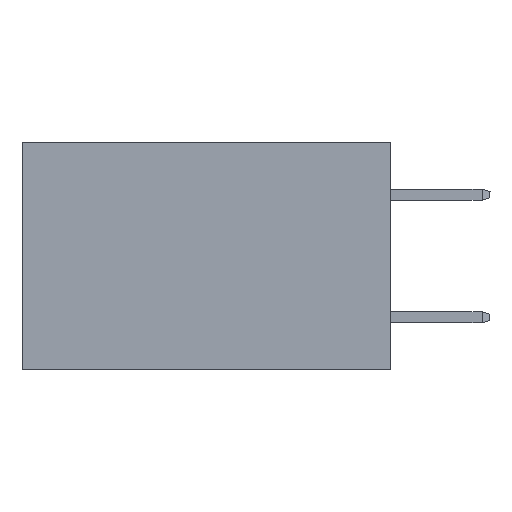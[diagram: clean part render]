
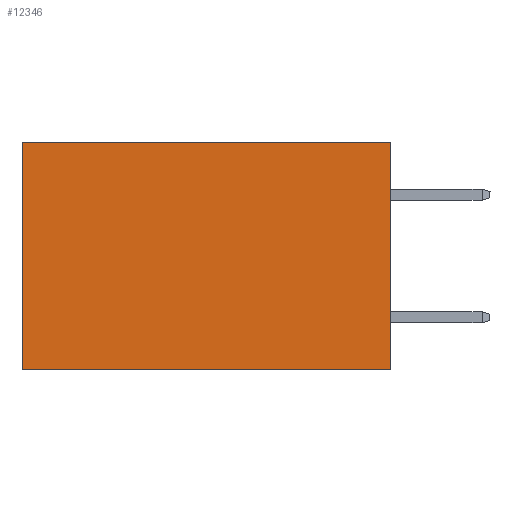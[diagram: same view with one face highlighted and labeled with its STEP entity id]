
A CAD part, left-side view. The second image highlights one B-rep face of the part: STEP entity #12346.
In plain terms, the highlighted planar face has unit normal (-1, 0, 0).
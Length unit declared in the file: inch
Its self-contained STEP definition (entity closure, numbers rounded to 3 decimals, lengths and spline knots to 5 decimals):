
#1113 = VERTEX_POINT ( 'NONE', #32478 ) ;
#1976 = VERTEX_POINT ( 'NONE', #24686 ) ;
#2902 = VECTOR ( 'NONE', #20083, 39.37008 ) ;
#5426 = CARTESIAN_POINT ( 'NONE',  ( 0.2875, 0.6, 0. ) ) ;
#5568 = DIRECTION ( 'NONE',  ( 0., 0., -1. ) ) ;
#6611 = EDGE_CURVE ( 'NONE', #1113, #8995, #24639, .T. ) ;
#7061 = DIRECTION ( 'NONE',  ( 0., 0., -1. ) ) ;
#8003 = LINE ( 'NONE', #25964, #29799 ) ;
#8931 = CARTESIAN_POINT ( 'NONE',  ( 0.2875, 0., 0. ) ) ;
#8995 = VERTEX_POINT ( 'NONE', #32847 ) ;
#9160 = EDGE_CURVE ( 'NONE', #16201, #8995, #28590, .T. ) ;
#9672 = EDGE_CURVE ( 'NONE', #1976, #1113, #33399, .T. ) ;
#11217 = AXIS2_PLACEMENT_3D ( 'NONE', #8931, #31268, #5568 ) ;
#11242 = CARTESIAN_POINT ( 'NONE',  ( 0.2875, 0.6, 0. ) ) ;
#12346 = ADVANCED_FACE ( 'NONE', ( #15435 ), #24149, .F. ) ;
#15188 = VECTOR ( 'NONE', #31355, 39.37008 ) ;
#15435 = FACE_OUTER_BOUND ( 'NONE', #21912, .T. ) ;
#16114 = EDGE_CURVE ( 'NONE', #1976, #16201, #8003, .T. ) ;
#16201 = VERTEX_POINT ( 'NONE', #5426 ) ;
#17057 = ORIENTED_EDGE ( 'NONE', *, *, #9672, .F. ) ;
#17547 = ORIENTED_EDGE ( 'NONE', *, *, #9160, .T. ) ;
#17922 = CARTESIAN_POINT ( 'NONE',  ( 0.2875, 0., 0. ) ) ;
#20083 = DIRECTION ( 'NONE',  ( 0., 1., 0. ) ) ;
#21912 = EDGE_LOOP ( 'NONE', ( #17547, #30310, #17057, #29388 ) ) ;
#23240 = DIRECTION ( 'NONE',  ( 0., 1., 0. ) ) ;
#24149 = PLANE ( 'NONE',  #11217 ) ;
#24639 = LINE ( 'NONE', #25291, #2902 ) ;
#24686 = CARTESIAN_POINT ( 'NONE',  ( 0.2875, 0., 0. ) ) ;
#25291 = CARTESIAN_POINT ( 'NONE',  ( 0.2875, 0., -0.37 ) ) ;
#25964 = CARTESIAN_POINT ( 'NONE',  ( 0.2875, 0., 0. ) ) ;
#28590 = LINE ( 'NONE', #11242, #31002 ) ;
#29388 = ORIENTED_EDGE ( 'NONE', *, *, #16114, .T. ) ;
#29799 = VECTOR ( 'NONE', #23240, 39.37008 ) ;
#30310 = ORIENTED_EDGE ( 'NONE', *, *, #6611, .F. ) ;
#31002 = VECTOR ( 'NONE', #7061, 39.37008 ) ;
#31268 = DIRECTION ( 'NONE',  ( 1., 0., 0. ) ) ;
#31355 = DIRECTION ( 'NONE',  ( 0., 0., -1. ) ) ;
#32478 = CARTESIAN_POINT ( 'NONE',  ( 0.2875, 0., -0.37 ) ) ;
#32847 = CARTESIAN_POINT ( 'NONE',  ( 0.2875, 0.6, -0.37 ) ) ;
#33399 = LINE ( 'NONE', #17922, #15188 ) ;
